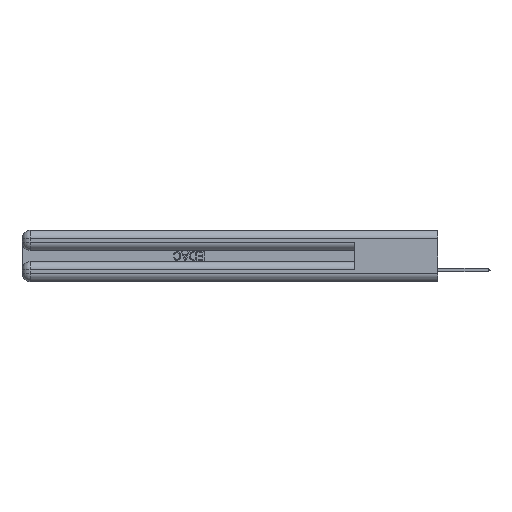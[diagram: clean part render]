
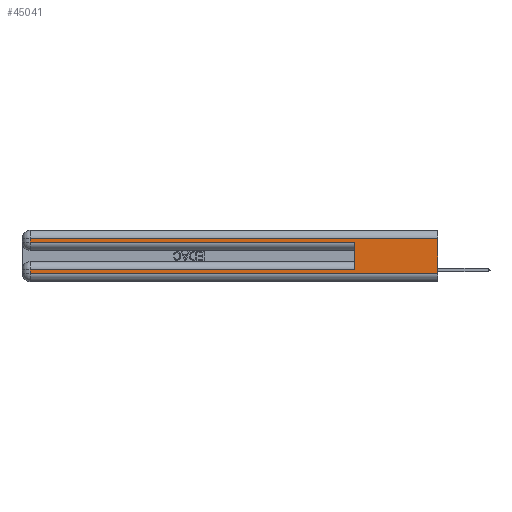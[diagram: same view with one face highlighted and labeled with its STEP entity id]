
A CAD part, left-side view. The second image highlights one B-rep face of the part: STEP entity #45041.
In plain terms, the highlighted planar face has unit normal (-1, 0, 0).
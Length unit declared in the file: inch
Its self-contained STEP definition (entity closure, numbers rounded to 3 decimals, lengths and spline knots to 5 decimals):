
#198 = ORIENTED_EDGE ( 'NONE', *, *, #29469, .T. ) ;
#1105 = VECTOR ( 'NONE', #6705, 39.37008 ) ;
#2131 = LINE ( 'NONE', #39722, #23646 ) ;
#2892 = DIRECTION ( 'NONE',  ( 0., 0., 1. ) ) ;
#2940 = LINE ( 'NONE', #15539, #11196 ) ;
#3813 = VERTEX_POINT ( 'NONE', #21799 ) ;
#4003 = CARTESIAN_POINT ( 'NONE',  ( 0., 0., 0.37 ) ) ;
#4275 = ORIENTED_EDGE ( 'NONE', *, *, #10452, .T. ) ;
#4801 = CARTESIAN_POINT ( 'NONE',  ( 0., 0., 0.06 ) ) ;
#4979 = CARTESIAN_POINT ( 'NONE',  ( 0., 0., 0.31 ) ) ;
#5948 = ORIENTED_EDGE ( 'NONE', *, *, #28551, .T. ) ;
#6705 = DIRECTION ( 'NONE',  ( 0., 0., -1. ) ) ;
#7278 = DIRECTION ( 'NONE',  ( 0., -1., 0. ) ) ;
#7504 = CARTESIAN_POINT ( 'NONE',  ( 0., 0.6, 0.145 ) ) ;
#8083 = EDGE_CURVE ( 'NONE', #38687, #29195, #10536, .T. ) ;
#10249 = CARTESIAN_POINT ( 'NONE',  ( 0., 2.94, 0.37 ) ) ;
#10452 = EDGE_CURVE ( 'NONE', #11919, #29195, #44883, .T. ) ;
#10536 = LINE ( 'NONE', #24137, #26318 ) ;
#11196 = VECTOR ( 'NONE', #29698, 39.37008 ) ;
#11500 = PLANE ( 'NONE',  #23965 ) ;
#11919 = VERTEX_POINT ( 'NONE', #37842 ) ;
#11936 = LINE ( 'NONE', #10249, #1105 ) ;
#14663 = EDGE_LOOP ( 'NONE', ( #16691, #198, #5948, #35348, #24754, #27603, #22895, #4275 ) ) ;
#15454 = CARTESIAN_POINT ( 'NONE',  ( 0., 0., 0.085 ) ) ;
#15539 = CARTESIAN_POINT ( 'NONE',  ( 0., 0., 0.31 ) ) ;
#15875 = LINE ( 'NONE', #7504, #39828 ) ;
#15927 = DIRECTION ( 'NONE',  ( 0., 0., -1. ) ) ;
#16175 = CARTESIAN_POINT ( 'NONE',  ( 0., 0.6, 0.085 ) ) ;
#16691 = ORIENTED_EDGE ( 'NONE', *, *, #8083, .F. ) ;
#20281 = CARTESIAN_POINT ( 'NONE',  ( 0., 2.94, 0.31 ) ) ;
#21775 = CARTESIAN_POINT ( 'NONE',  ( 0., 2.94, 0.085 ) ) ;
#21799 = CARTESIAN_POINT ( 'NONE',  ( 0., 2.94, 0.285 ) ) ;
#21824 = CARTESIAN_POINT ( 'NONE',  ( 0., 2.94, 0.37 ) ) ;
#22895 = ORIENTED_EDGE ( 'NONE', *, *, #44398, .T. ) ;
#23646 = VECTOR ( 'NONE', #7278, 39.37008 ) ;
#23668 = DIRECTION ( 'NONE',  ( 1., 0., 0. ) ) ;
#23965 = AXIS2_PLACEMENT_3D ( 'NONE', #4003, #23668, #15927 ) ;
#24137 = CARTESIAN_POINT ( 'NONE',  ( 0., 0., 0.37 ) ) ;
#24754 = ORIENTED_EDGE ( 'NONE', *, *, #40766, .F. ) ;
#24796 = DIRECTION ( 'NONE',  ( 0., 0., -1. ) ) ;
#25343 = EDGE_CURVE ( 'NONE', #3813, #52257, #2131, .T. ) ;
#26318 = VECTOR ( 'NONE', #24796, 39.37008 ) ;
#27603 = ORIENTED_EDGE ( 'NONE', *, *, #36511, .T. ) ;
#28168 = VECTOR ( 'NONE', #47980, 39.37008 ) ;
#28281 = LINE ( 'NONE', #21824, #43428 ) ;
#28551 = EDGE_CURVE ( 'NONE', #40331, #3813, #28281, .T. ) ;
#29195 = VERTEX_POINT ( 'NONE', #4801 ) ;
#29469 = EDGE_CURVE ( 'NONE', #38687, #40331, #2940, .T. ) ;
#29698 = DIRECTION ( 'NONE',  ( 0., 1., 0. ) ) ;
#32858 = VERTEX_POINT ( 'NONE', #21775 ) ;
#35348 = ORIENTED_EDGE ( 'NONE', *, *, #25343, .T. ) ;
#35502 = VECTOR ( 'NONE', #39246, 39.37008 ) ;
#36390 = FACE_OUTER_BOUND ( 'NONE', #14663, .T. ) ;
#36511 = EDGE_CURVE ( 'NONE', #50874, #32858, #42685, .T. ) ;
#37842 = CARTESIAN_POINT ( 'NONE',  ( 0., 2.94, 0.06 ) ) ;
#38555 = DIRECTION ( 'NONE',  ( 0., 0., -1. ) ) ;
#38687 = VERTEX_POINT ( 'NONE', #4979 ) ;
#39246 = DIRECTION ( 'NONE',  ( 0., -1., 0. ) ) ;
#39722 = CARTESIAN_POINT ( 'NONE',  ( 0., 0., 0.285 ) ) ;
#39828 = VECTOR ( 'NONE', #2892, 39.37008 ) ;
#40331 = VERTEX_POINT ( 'NONE', #20281 ) ;
#40766 = EDGE_CURVE ( 'NONE', #50874, #52257, #15875, .T. ) ;
#42685 = LINE ( 'NONE', #15454, #28168 ) ;
#43428 = VECTOR ( 'NONE', #38555, 39.37008 ) ;
#44398 = EDGE_CURVE ( 'NONE', #32858, #11919, #11936, .T. ) ;
#44883 = LINE ( 'NONE', #47644, #35502 ) ;
#45041 = ADVANCED_FACE ( 'NONE', ( #36390 ), #11500, .F. ) ;
#47644 = CARTESIAN_POINT ( 'NONE',  ( 0., 0., 0.06 ) ) ;
#47980 = DIRECTION ( 'NONE',  ( 0., 1., 0. ) ) ;
#50098 = CARTESIAN_POINT ( 'NONE',  ( 0., 0.6, 0.285 ) ) ;
#50874 = VERTEX_POINT ( 'NONE', #16175 ) ;
#52257 = VERTEX_POINT ( 'NONE', #50098 ) ;
